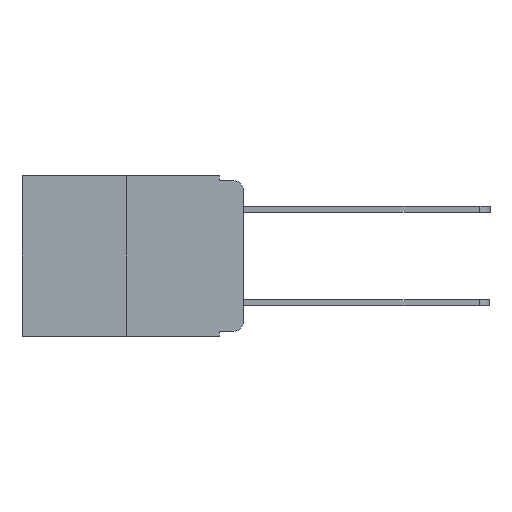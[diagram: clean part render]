
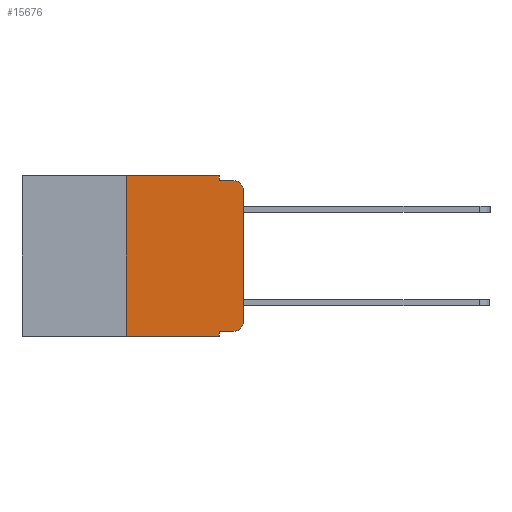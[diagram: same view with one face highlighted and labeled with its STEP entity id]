
A CAD part, left-side view. The second image highlights one B-rep face of the part: STEP entity #15676.
In plain terms, the highlighted planar face has unit normal (-1, 0, 0).
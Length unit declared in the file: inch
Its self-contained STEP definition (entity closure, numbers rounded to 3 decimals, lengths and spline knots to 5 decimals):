
#176 = DIRECTION ( 'NONE',  ( 0., 0., -1. ) ) ;
#559 = VECTOR ( 'NONE', #16298, 39.37008 ) ;
#1255 = VERTEX_POINT ( 'NONE', #18125 ) ;
#1340 = VERTEX_POINT ( 'NONE', #18332 ) ;
#1818 = EDGE_CURVE ( 'NONE', #17723, #1255, #15582, .T. ) ;
#2368 = CARTESIAN_POINT ( 'NONE',  ( 0., 0.473, 0. ) ) ;
#2391 = DIRECTION ( 'NONE',  ( 0., -1., 0. ) ) ;
#2676 = AXIS2_PLACEMENT_3D ( 'NONE', #13695, #5014, #17090 ) ;
#3137 = PLANE ( 'NONE',  #2676 ) ;
#3632 = VECTOR ( 'NONE', #7731, 39.37008 ) ;
#3781 = ORIENTED_EDGE ( 'NONE', *, *, #16599, .T. ) ;
#4035 = ORIENTED_EDGE ( 'NONE', *, *, #14440, .F. ) ;
#4151 = DIRECTION ( 'NONE',  ( 0., 0., -1. ) ) ;
#4367 = VECTOR ( 'NONE', #11381, 39.37008 ) ;
#4574 = DIRECTION ( 'NONE',  ( 0., 0., -1. ) ) ;
#4867 = ORIENTED_EDGE ( 'NONE', *, *, #18809, .F. ) ;
#5014 = DIRECTION ( 'NONE',  ( 1., 0., 0. ) ) ;
#6117 = CARTESIAN_POINT ( 'NONE',  ( 0., 0.25, 0. ) ) ;
#6358 = VECTOR ( 'NONE', #4151, 39.37008 ) ;
#6742 = LINE ( 'NONE', #7998, #15423 ) ;
#6887 = LINE ( 'NONE', #21563, #10986 ) ;
#7068 = CARTESIAN_POINT ( 'NONE',  ( 0., 0., -0.03 ) ) ;
#7105 = VERTEX_POINT ( 'NONE', #20345 ) ;
#7346 = ORIENTED_EDGE ( 'NONE', *, *, #1818, .F. ) ;
#7376 = CARTESIAN_POINT ( 'NONE',  ( 0., 0.051, -0.333 ) ) ;
#7536 = CARTESIAN_POINT ( 'NONE',  ( 0., 0.051, 0. ) ) ;
#7731 = DIRECTION ( 'NONE',  ( 0., 0., 1. ) ) ;
#7939 = CARTESIAN_POINT ( 'NONE',  ( 0., 0.02, -0.03 ) ) ;
#7998 = CARTESIAN_POINT ( 'NONE',  ( 0., 0.051, 0. ) ) ;
#8835 = LINE ( 'NONE', #16331, #3632 ) ;
#9353 = EDGE_CURVE ( 'NONE', #11723, #15973, #18635, .T. ) ;
#9603 = CARTESIAN_POINT ( 'NONE',  ( 0., 0.051, -0.01 ) ) ;
#9684 = DIRECTION ( 'NONE',  ( 0., 0., -1. ) ) ;
#9720 = VECTOR ( 'NONE', #2391, 39.37008 ) ;
#10282 = VERTEX_POINT ( 'NONE', #9603 ) ;
#10350 = ORIENTED_EDGE ( 'NONE', *, *, #20104, .T. ) ;
#10785 = VERTEX_POINT ( 'NONE', #7536 ) ;
#10851 = DIRECTION ( 'NONE',  ( -1., 0., 0. ) ) ;
#10873 = ORIENTED_EDGE ( 'NONE', *, *, #18937, .F. ) ;
#10986 = VECTOR ( 'NONE', #14911, 39.37008 ) ;
#11225 = VECTOR ( 'NONE', #14483, 39.37008 ) ;
#11240 = VERTEX_POINT ( 'NONE', #18959 ) ;
#11381 = DIRECTION ( 'NONE',  ( 0., 0., 1. ) ) ;
#11723 = VERTEX_POINT ( 'NONE', #20173 ) ;
#11755 = LINE ( 'NONE', #12745, #11225 ) ;
#11845 = EDGE_LOOP ( 'NONE', ( #19621, #12765, #4035, #10873, #4867, #21226, #10350, #7346, #3781, #22006 ) ) ;
#12127 = EDGE_CURVE ( 'NONE', #21027, #1340, #22415, .T. ) ;
#12745 = CARTESIAN_POINT ( 'NONE',  ( 0., 0.051, -0.333 ) ) ;
#12765 = ORIENTED_EDGE ( 'NONE', *, *, #12127, .T. ) ;
#13695 = CARTESIAN_POINT ( 'NONE',  ( 0., 0.473, 0. ) ) ;
#13723 = EDGE_CURVE ( 'NONE', #11240, #21027, #8835, .T. ) ;
#14084 = CIRCLE ( 'NONE', #20495, 0.02 ) ;
#14332 = LINE ( 'NONE', #18005, #9720 ) ;
#14440 = EDGE_CURVE ( 'NONE', #10282, #1340, #6887, .T. ) ;
#14483 = DIRECTION ( 'NONE',  ( 0., -1., 0. ) ) ;
#14588 = CARTESIAN_POINT ( 'NONE',  ( 0., 0.051, 0. ) ) ;
#14911 = DIRECTION ( 'NONE',  ( 0., -1., 0. ) ) ;
#15423 = VECTOR ( 'NONE', #4574, 39.37008 ) ;
#15582 = LINE ( 'NONE', #14588, #6358 ) ;
#15676 = ADVANCED_FACE ( 'NONE', ( #18719 ), #3137, .F. ) ;
#15705 = AXIS2_PLACEMENT_3D ( 'NONE', #7939, #19873, #9684 ) ;
#15973 = VERTEX_POINT ( 'NONE', #19553 ) ;
#16298 = DIRECTION ( 'NONE',  ( 0., -1., 0. ) ) ;
#16331 = CARTESIAN_POINT ( 'NONE',  ( 0., 0., 0. ) ) ;
#16599 = EDGE_CURVE ( 'NONE', #17723, #7105, #11755, .T. ) ;
#17090 = DIRECTION ( 'NONE',  ( 0., 0., -1. ) ) ;
#17723 = VERTEX_POINT ( 'NONE', #7376 ) ;
#18005 = CARTESIAN_POINT ( 'NONE',  ( 0., 0.473, -0.343 ) ) ;
#18125 = CARTESIAN_POINT ( 'NONE',  ( 0., 0.051, -0.343 ) ) ;
#18332 = CARTESIAN_POINT ( 'NONE',  ( 0., 0.02, -0.01 ) ) ;
#18635 = LINE ( 'NONE', #6117, #4367 ) ;
#18719 = FACE_OUTER_BOUND ( 'NONE', #11845, .T. ) ;
#18809 = EDGE_CURVE ( 'NONE', #15973, #10785, #19082, .T. ) ;
#18937 = EDGE_CURVE ( 'NONE', #10785, #10282, #6742, .T. ) ;
#18959 = CARTESIAN_POINT ( 'NONE',  ( 0., 0., -0.313 ) ) ;
#19082 = LINE ( 'NONE', #2368, #559 ) ;
#19553 = CARTESIAN_POINT ( 'NONE',  ( 0., 0.25, 0. ) ) ;
#19621 = ORIENTED_EDGE ( 'NONE', *, *, #13723, .T. ) ;
#19873 = DIRECTION ( 'NONE',  ( -1., 0., 0. ) ) ;
#19945 = EDGE_CURVE ( 'NONE', #7105, #11240, #14084, .T. ) ;
#20104 = EDGE_CURVE ( 'NONE', #11723, #1255, #14332, .T. ) ;
#20173 = CARTESIAN_POINT ( 'NONE',  ( 0., 0.25, -0.343 ) ) ;
#20345 = CARTESIAN_POINT ( 'NONE',  ( 0., 0.02, -0.333 ) ) ;
#20495 = AXIS2_PLACEMENT_3D ( 'NONE', #20993, #10851, #176 ) ;
#20993 = CARTESIAN_POINT ( 'NONE',  ( 0., 0.02, -0.313 ) ) ;
#21027 = VERTEX_POINT ( 'NONE', #7068 ) ;
#21226 = ORIENTED_EDGE ( 'NONE', *, *, #9353, .F. ) ;
#21563 = CARTESIAN_POINT ( 'NONE',  ( 0., 0.051, -0.01 ) ) ;
#22006 = ORIENTED_EDGE ( 'NONE', *, *, #19945, .T. ) ;
#22415 = CIRCLE ( 'NONE', #15705, 0.02 ) ;
